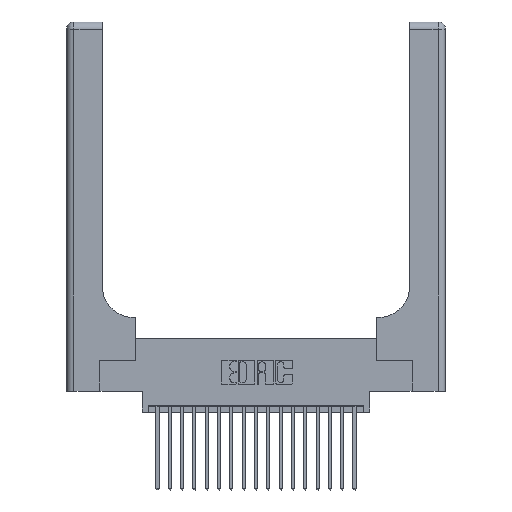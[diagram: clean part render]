
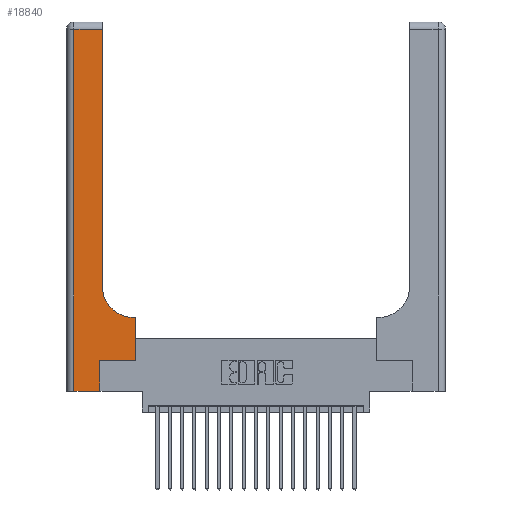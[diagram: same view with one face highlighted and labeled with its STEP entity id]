
A CAD part, top view. The second image highlights one B-rep face of the part: STEP entity #18840.
In plain terms, the highlighted planar face has unit normal (0, 0, 1).
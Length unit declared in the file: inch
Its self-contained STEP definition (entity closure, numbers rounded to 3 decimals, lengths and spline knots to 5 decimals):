
#152 = VERTEX_POINT ( 'NONE', #552 ) ;
#321 = CARTESIAN_POINT ( 'NONE',  ( 0.06, 2.94, 0.37 ) ) ;
#552 = CARTESIAN_POINT ( 'NONE',  ( 0.5585, 0.25, 0.37 ) ) ;
#1138 = CARTESIAN_POINT ( 'NONE',  ( 0.06, 3., 0.37 ) ) ;
#1315 = ORIENTED_EDGE ( 'NONE', *, *, #13323, .T. ) ;
#1493 = DIRECTION ( 'NONE',  ( 0., 1., 0. ) ) ;
#1964 = ORIENTED_EDGE ( 'NONE', *, *, #18993, .T. ) ;
#2490 = LINE ( 'NONE', #12401, #19980 ) ;
#2549 = VECTOR ( 'NONE', #16261, 39.37008 ) ;
#2584 = DIRECTION ( 'NONE',  ( 0., 0., -1. ) ) ;
#2660 = CARTESIAN_POINT ( 'NONE',  ( 0., 2.94, 0.37 ) ) ;
#3072 = ORIENTED_EDGE ( 'NONE', *, *, #13783, .T. ) ;
#3100 = EDGE_LOOP ( 'NONE', ( #1964, #1315, #10476, #8903, #3072, #5963, #9166, #20073, #19139 ) ) ;
#4565 = EDGE_CURVE ( 'NONE', #13223, #18118, #2490, .T. ) ;
#4697 = LINE ( 'NONE', #20910, #13615 ) ;
#5060 = LINE ( 'NONE', #13801, #5614 ) ;
#5329 = CARTESIAN_POINT ( 'NONE',  ( 0.06, 0., 0.37 ) ) ;
#5334 = AXIS2_PLACEMENT_3D ( 'NONE', #19555, #21246, #11094 ) ;
#5446 = DIRECTION ( 'NONE',  ( 1., 0., 0. ) ) ;
#5455 = CARTESIAN_POINT ( 'NONE',  ( 0.269, 0., 0.37 ) ) ;
#5614 = VECTOR ( 'NONE', #5446, 39.37008 ) ;
#5774 = DIRECTION ( 'NONE',  ( -1., 0., 0. ) ) ;
#5809 = DIRECTION ( 'NONE',  ( 1., 0., 0. ) ) ;
#5963 = ORIENTED_EDGE ( 'NONE', *, *, #19806, .T. ) ;
#6360 = VECTOR ( 'NONE', #7242, 39.37008 ) ;
#6740 = EDGE_CURVE ( 'NONE', #18118, #18056, #10096, .T. ) ;
#7242 = DIRECTION ( 'NONE',  ( 0., 1., 0. ) ) ;
#7657 = VECTOR ( 'NONE', #1493, 39.37008 ) ;
#7664 = LINE ( 'NONE', #2660, #2549 ) ;
#7764 = PLANE ( 'NONE',  #5334 ) ;
#8075 = LINE ( 'NONE', #21627, #11953 ) ;
#8250 = VERTEX_POINT ( 'NONE', #5329 ) ;
#8357 = VERTEX_POINT ( 'NONE', #321 ) ;
#8903 = ORIENTED_EDGE ( 'NONE', *, *, #21998, .T. ) ;
#9124 = VECTOR ( 'NONE', #14795, 39.37008 ) ;
#9166 = ORIENTED_EDGE ( 'NONE', *, *, #9741, .T. ) ;
#9678 = EDGE_CURVE ( 'NONE', #8357, #8250, #18125, .T. ) ;
#9741 = EDGE_CURVE ( 'NONE', #152, #13223, #8075, .T. ) ;
#10001 = CARTESIAN_POINT ( 'NONE',  ( 0.2915, 3., 0.37 ) ) ;
#10096 = CIRCLE ( 'NONE', #15271, 0.25 ) ;
#10432 = CARTESIAN_POINT ( 'NONE',  ( 0.5585, 0.6, 0.37 ) ) ;
#10476 = ORIENTED_EDGE ( 'NONE', *, *, #9678, .T. ) ;
#11094 = DIRECTION ( 'NONE',  ( -1., 0., 0. ) ) ;
#11821 = LINE ( 'NONE', #5455, #6360 ) ;
#11953 = VECTOR ( 'NONE', #20010, 39.37008 ) ;
#12049 = LINE ( 'NONE', #10001, #7657 ) ;
#12401 = CARTESIAN_POINT ( 'NONE',  ( 0.2915, 0.6, 0.37 ) ) ;
#12695 = CARTESIAN_POINT ( 'NONE',  ( 0.5415, 0.85, 0.37 ) ) ;
#13223 = VERTEX_POINT ( 'NONE', #10432 ) ;
#13323 = EDGE_CURVE ( 'NONE', #14939, #8357, #7664, .T. ) ;
#13615 = VECTOR ( 'NONE', #5809, 39.37008 ) ;
#13783 = EDGE_CURVE ( 'NONE', #14789, #14945, #11821, .T. ) ;
#13801 = CARTESIAN_POINT ( 'NONE',  ( 0., 0., 0.37 ) ) ;
#14468 = DIRECTION ( 'NONE',  ( 1., 0., 0. ) ) ;
#14789 = VERTEX_POINT ( 'NONE', #19946 ) ;
#14795 = DIRECTION ( 'NONE',  ( 0., -1., 0. ) ) ;
#14939 = VERTEX_POINT ( 'NONE', #21911 ) ;
#14945 = VERTEX_POINT ( 'NONE', #18650 ) ;
#15271 = AXIS2_PLACEMENT_3D ( 'NONE', #12695, #2584, #14468 ) ;
#16058 = CARTESIAN_POINT ( 'NONE',  ( 0.5415, 0.6, 0.37 ) ) ;
#16261 = DIRECTION ( 'NONE',  ( -1., 0., 0. ) ) ;
#17571 = CARTESIAN_POINT ( 'NONE',  ( 0.2915, 0.85, 0.37 ) ) ;
#18056 = VERTEX_POINT ( 'NONE', #17571 ) ;
#18118 = VERTEX_POINT ( 'NONE', #16058 ) ;
#18125 = LINE ( 'NONE', #1138, #9124 ) ;
#18650 = CARTESIAN_POINT ( 'NONE',  ( 0.269, 0.25, 0.37 ) ) ;
#18840 = ADVANCED_FACE ( 'NONE', ( #19272 ), #7764, .F. ) ;
#18993 = EDGE_CURVE ( 'NONE', #18056, #14939, #12049, .T. ) ;
#19139 = ORIENTED_EDGE ( 'NONE', *, *, #6740, .T. ) ;
#19272 = FACE_OUTER_BOUND ( 'NONE', #3100, .T. ) ;
#19555 = CARTESIAN_POINT ( 'NONE',  ( 0., 3., 0.37 ) ) ;
#19806 = EDGE_CURVE ( 'NONE', #14945, #152, #4697, .T. ) ;
#19946 = CARTESIAN_POINT ( 'NONE',  ( 0.269, 0., 0.37 ) ) ;
#19980 = VECTOR ( 'NONE', #5774, 39.37008 ) ;
#20010 = DIRECTION ( 'NONE',  ( 0., 1., 0. ) ) ;
#20073 = ORIENTED_EDGE ( 'NONE', *, *, #4565, .T. ) ;
#20910 = CARTESIAN_POINT ( 'NONE',  ( 0.269, 0.25, 0.37 ) ) ;
#21246 = DIRECTION ( 'NONE',  ( 0., 0., -1. ) ) ;
#21627 = CARTESIAN_POINT ( 'NONE',  ( 0.5585, 0.25, 0.37 ) ) ;
#21911 = CARTESIAN_POINT ( 'NONE',  ( 0.2915, 2.94, 0.37 ) ) ;
#21998 = EDGE_CURVE ( 'NONE', #8250, #14789, #5060, .T. ) ;
